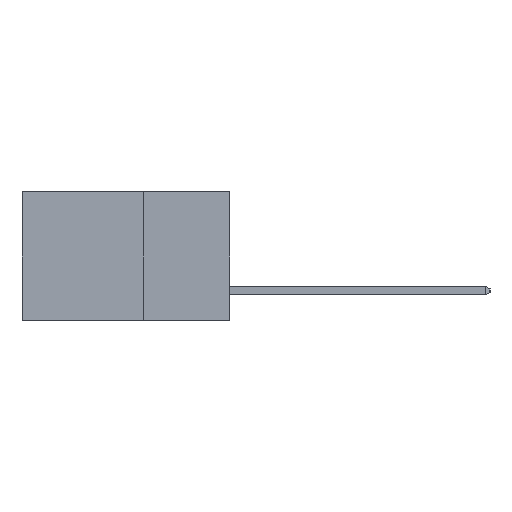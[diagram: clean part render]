
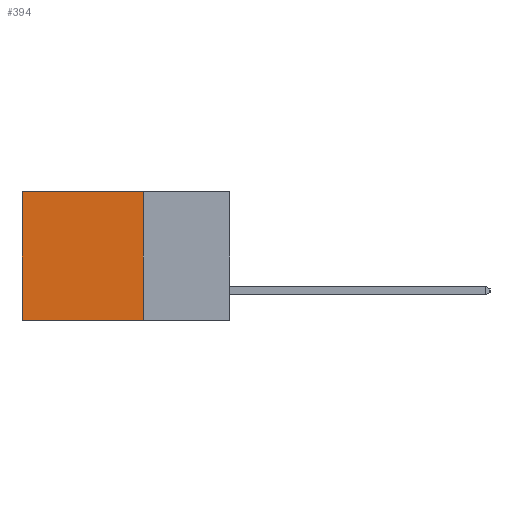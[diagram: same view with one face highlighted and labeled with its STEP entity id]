
A CAD part, left-side view. The second image highlights one B-rep face of the part: STEP entity #394.
In plain terms, the highlighted planar face has unit normal (-1, 0, 0).
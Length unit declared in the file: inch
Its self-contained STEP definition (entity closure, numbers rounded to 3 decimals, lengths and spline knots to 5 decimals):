
#346 = EDGE_CURVE ( 'NONE', #9224, #2500, #462, .T. ) ;
#394 = ADVANCED_FACE ( 'NONE', ( #7308 ), #11274, .F. ) ;
#462 = LINE ( 'NONE', #5285, #7927 ) ;
#807 = CARTESIAN_POINT ( 'NONE',  ( 0.2615, 0.25, -0.37 ) ) ;
#829 = CARTESIAN_POINT ( 'NONE',  ( 0.2615, 0.25, -0.37 ) ) ;
#1098 = EDGE_CURVE ( 'NONE', #9224, #10512, #9406, .T. ) ;
#1235 = VECTOR ( 'NONE', #11450, 39.37008 ) ;
#1954 = DIRECTION ( 'NONE',  ( 0., 0., -1. ) ) ;
#2003 = DIRECTION ( 'NONE',  ( 1., 0., 0. ) ) ;
#2500 = VERTEX_POINT ( 'NONE', #4922 ) ;
#2699 = CARTESIAN_POINT ( 'NONE',  ( 0.2615, 0.6, -0.37 ) ) ;
#3877 = LINE ( 'NONE', #829, #1235 ) ;
#4624 = CARTESIAN_POINT ( 'NONE',  ( 0.2615, 0.25, 0. ) ) ;
#4922 = CARTESIAN_POINT ( 'NONE',  ( 0.2615, 0.6, 0. ) ) ;
#5033 = ORIENTED_EDGE ( 'NONE', *, *, #6598, .T. ) ;
#5285 = CARTESIAN_POINT ( 'NONE',  ( 0.2615, 0.25, 0. ) ) ;
#5464 = AXIS2_PLACEMENT_3D ( 'NONE', #11131, #2003, #1954 ) ;
#6429 = VERTEX_POINT ( 'NONE', #7272 ) ;
#6587 = ORIENTED_EDGE ( 'NONE', *, *, #346, .T. ) ;
#6598 = EDGE_CURVE ( 'NONE', #2500, #6429, #9797, .T. ) ;
#7123 = VECTOR ( 'NONE', #9399, 39.37008 ) ;
#7272 = CARTESIAN_POINT ( 'NONE',  ( 0.2615, 0.6, -0.37 ) ) ;
#7308 = FACE_OUTER_BOUND ( 'NONE', #9484, .T. ) ;
#7336 = EDGE_CURVE ( 'NONE', #10512, #6429, #3877, .T. ) ;
#7927 = VECTOR ( 'NONE', #8307, 39.37008 ) ;
#8307 = DIRECTION ( 'NONE',  ( 0., 1., 0. ) ) ;
#9224 = VERTEX_POINT ( 'NONE', #4624 ) ;
#9361 = CARTESIAN_POINT ( 'NONE',  ( 0.2615, 0.25, -0.37 ) ) ;
#9399 = DIRECTION ( 'NONE',  ( 0., 0., -1. ) ) ;
#9406 = LINE ( 'NONE', #807, #7123 ) ;
#9484 = EDGE_LOOP ( 'NONE', ( #5033, #10676, #10999, #6587 ) ) ;
#9797 = LINE ( 'NONE', #2699, #11935 ) ;
#10443 = DIRECTION ( 'NONE',  ( 0., 0., -1. ) ) ;
#10512 = VERTEX_POINT ( 'NONE', #9361 ) ;
#10676 = ORIENTED_EDGE ( 'NONE', *, *, #7336, .F. ) ;
#10999 = ORIENTED_EDGE ( 'NONE', *, *, #1098, .F. ) ;
#11131 = CARTESIAN_POINT ( 'NONE',  ( 0.2615, 0.25, -0.37 ) ) ;
#11274 = PLANE ( 'NONE',  #5464 ) ;
#11450 = DIRECTION ( 'NONE',  ( 0., 1., 0. ) ) ;
#11935 = VECTOR ( 'NONE', #10443, 39.37008 ) ;
